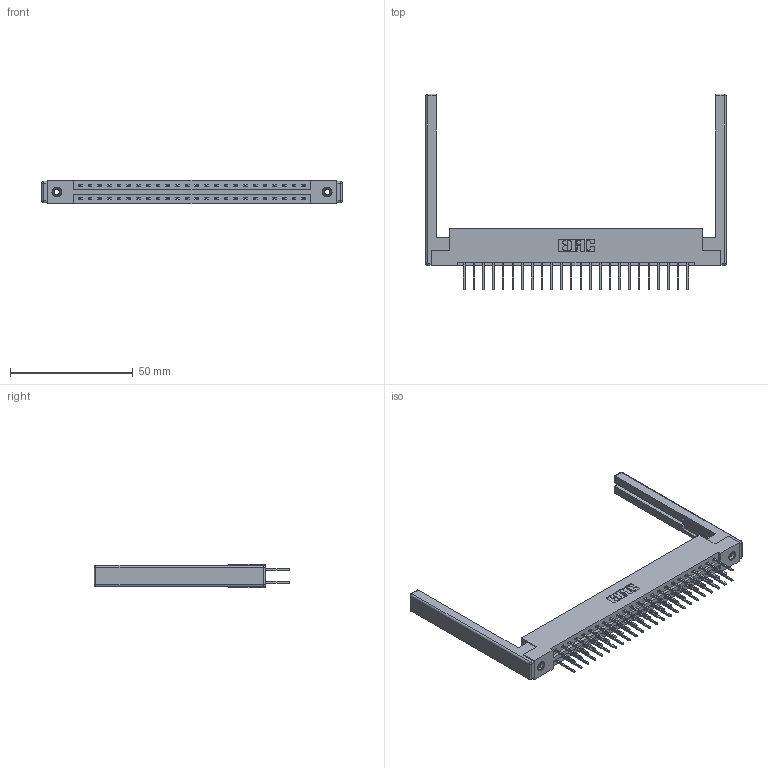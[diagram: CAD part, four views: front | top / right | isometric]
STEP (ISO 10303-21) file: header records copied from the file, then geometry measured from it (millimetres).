
FILE_DESCRIPTION (( 'STEP AP203' ), '1' );
FILE_NAME ('387-048-523-268.STEP', '2019-10-18T09:19:11', ( '' ), ( '' ), 'SwSTEP 2.0', 'SolidWorks 2016', '' );
FILE_SCHEMA (( 'CONFIG_CONTROL_DESIGN' ));
Length unit declared in the file: inch
Products named in the file (5): 345-292-001_345-293-123; 345-250-001_345-250-001-102; 387-048-523-268; 307-220-068; 337 Part_Flush Mounting Lugs - 0.156 Dia-TI
Assembly tree (53 placements, depth 2):
  387-048-523-268
    337 Part_Flush Mounting Lugs - 0.156 Dia-TI
    345-292-001_345-293-123  x48
    345-250-001_345-250-001-102  x2
    307-220-068  x2
Bounding box: 122.53 x 79.89 x 9.4 mm (x, y, z)
Volume: 17156.7 mm3; surface area: 18765.8 mm2
Topology: 53 solids, 53 shells, 2860 faces, 8429 edges, 5534 vertices
Faces by surface type: plane 1982, cylinder 854, cone 12, sphere 8, torus 4
Entity records: 23714 total; most frequent: CARTESIAN_POINT 3975, ORIENTED_EDGE 3900, DIRECTION 3484, EDGE_CURVE 1950, VECTOR 1772, LINE 1772, VERTEX_POINT 1290, AXIS2_PLACEMENT_3D 856
